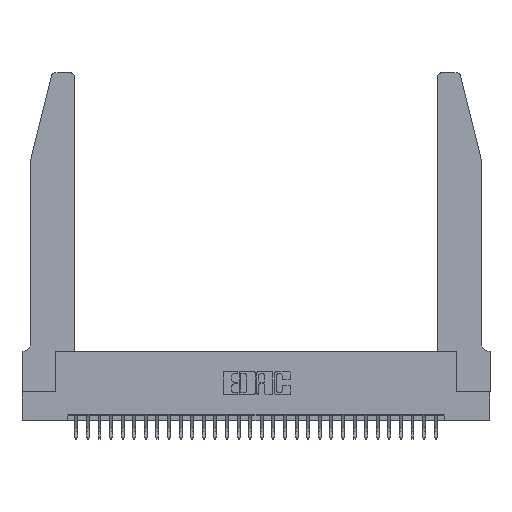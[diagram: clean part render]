
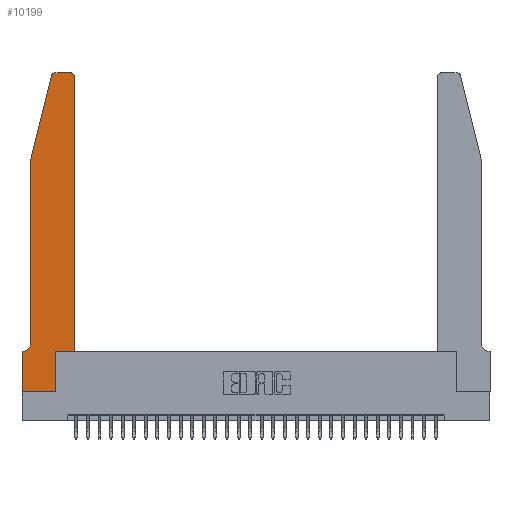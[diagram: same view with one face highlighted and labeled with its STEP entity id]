
A CAD part, top view. The second image highlights one B-rep face of the part: STEP entity #10199.
In plain terms, the highlighted planar face has unit normal (0, 0, 1).
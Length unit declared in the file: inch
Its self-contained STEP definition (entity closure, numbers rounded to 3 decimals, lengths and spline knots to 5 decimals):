
#533 = VECTOR ( 'NONE', #2375, 39.37008 ) ;
#574 = CARTESIAN_POINT ( 'NONE',  ( 0.0755, 0.42, 0.37 ) ) ;
#1327 = DIRECTION ( 'NONE',  ( 0., 1., 0. ) ) ;
#1335 = ORIENTED_EDGE ( 'NONE', *, *, #5731, .T. ) ;
#1471 = CARTESIAN_POINT ( 'NONE',  ( 0.2865, 0., 0.37 ) ) ;
#2073 = CARTESIAN_POINT ( 'NONE',  ( 0.4205, 2.72, 0.37 ) ) ;
#2176 = DIRECTION ( 'NONE',  ( 1., 0., 0. ) ) ;
#2247 = VECTOR ( 'NONE', #13660, 39.37008 ) ;
#2375 = DIRECTION ( 'NONE',  ( -1., 0., 0. ) ) ;
#2538 = EDGE_CURVE ( 'NONE', #26263, #22320, #18626, .T. ) ;
#2676 = VERTEX_POINT ( 'NONE', #9555 ) ;
#2763 = EDGE_CURVE ( 'NONE', #28510, #29235, #20082, .T. ) ;
#2786 = CARTESIAN_POINT ( 'NONE',  ( 0.2865, 0.35, 0.37 ) ) ;
#2855 = DIRECTION ( 'NONE',  ( 0., 0., -1. ) ) ;
#3597 = DIRECTION ( 'NONE',  ( 0., 0., 1. ) ) ;
#4156 = ORIENTED_EDGE ( 'NONE', *, *, #24620, .T. ) ;
#4180 = DIRECTION ( 'NONE',  ( 0., -1., 0. ) ) ;
#4250 = CIRCLE ( 'NONE', #20334, 0.07 ) ;
#4786 = AXIS2_PLACEMENT_3D ( 'NONE', #2073, #19172, #2176 ) ;
#4988 = VERTEX_POINT ( 'NONE', #8752 ) ;
#5173 = EDGE_CURVE ( 'NONE', #7477, #20418, #11264, .T. ) ;
#5637 = VERTEX_POINT ( 'NONE', #574 ) ;
#5731 = EDGE_CURVE ( 'NONE', #23783, #26263, #29848, .T. ) ;
#6413 = ORIENTED_EDGE ( 'NONE', *, *, #5173, .T. ) ;
#6653 = FACE_OUTER_BOUND ( 'NONE', #22145, .T. ) ;
#7132 = DIRECTION ( 'NONE',  ( 0., 0., 1. ) ) ;
#7250 = DIRECTION ( 'NONE',  ( -1., 0., 0. ) ) ;
#7477 = VERTEX_POINT ( 'NONE', #23795 ) ;
#7527 = ORIENTED_EDGE ( 'NONE', *, *, #22625, .T. ) ;
#7638 = CARTESIAN_POINT ( 'NONE',  ( 0.0055, 0.42, 0.37 ) ) ;
#8357 = CARTESIAN_POINT ( 'NONE',  ( 0.0755, 2., 0.37 ) ) ;
#8752 = CARTESIAN_POINT ( 'NONE',  ( 0.0055, 0.35, 0.37 ) ) ;
#8838 = EDGE_CURVE ( 'NONE', #5637, #4988, #4250, .T. ) ;
#9555 = CARTESIAN_POINT ( 'NONE',  ( 0.284, 2.75, 0.37 ) ) ;
#9731 = VECTOR ( 'NONE', #10140, 39.37008 ) ;
#10005 = CARTESIAN_POINT ( 'NONE',  ( 0.284, 2.72, 0.37 ) ) ;
#10140 = DIRECTION ( 'NONE',  ( 1., 0., 0. ) ) ;
#10199 = ADVANCED_FACE ( 'NONE', ( #6653 ), #18576, .T. ) ;
#10532 = VECTOR ( 'NONE', #13680, 39.37008 ) ;
#10593 = ORIENTED_EDGE ( 'NONE', *, *, #11465, .T. ) ;
#11264 = LINE ( 'NONE', #26016, #16211 ) ;
#11465 = EDGE_CURVE ( 'NONE', #20418, #17329, #13440, .T. ) ;
#11520 = LINE ( 'NONE', #19045, #19884 ) ;
#13440 = LINE ( 'NONE', #16291, #14199 ) ;
#13589 = CARTESIAN_POINT ( 'NONE',  ( 0., 0.35, 0.37 ) ) ;
#13660 = DIRECTION ( 'NONE',  ( -0.239, -0.971, 0. ) ) ;
#13664 = CIRCLE ( 'NONE', #4786, 0.03 ) ;
#13680 = DIRECTION ( 'NONE',  ( 0., -1., 0. ) ) ;
#13976 = EDGE_CURVE ( 'NONE', #22320, #15473, #13664, .T. ) ;
#14199 = VECTOR ( 'NONE', #28607, 39.37008 ) ;
#14656 = EDGE_CURVE ( 'NONE', #2676, #28510, #14735, .T. ) ;
#14735 = CIRCLE ( 'NONE', #31254, 0.03 ) ;
#14776 = VECTOR ( 'NONE', #1327, 39.37008 ) ;
#15473 = VERTEX_POINT ( 'NONE', #25119 ) ;
#16211 = VECTOR ( 'NONE', #4180, 39.37008 ) ;
#16291 = CARTESIAN_POINT ( 'NONE',  ( 0., 0., 0.37 ) ) ;
#17114 = VECTOR ( 'NONE', #28820, 39.37008 ) ;
#17196 = DIRECTION ( 'NONE',  ( -1., 0., 0. ) ) ;
#17244 = ORIENTED_EDGE ( 'NONE', *, *, #13976, .T. ) ;
#17255 = ORIENTED_EDGE ( 'NONE', *, *, #14656, .T. ) ;
#17329 = VERTEX_POINT ( 'NONE', #1471 ) ;
#17767 = CARTESIAN_POINT ( 'NONE',  ( 0.4505, 0.35, 0.37 ) ) ;
#18576 = PLANE ( 'NONE',  #26230 ) ;
#18626 = LINE ( 'NONE', #17767, #14776 ) ;
#18645 = ORIENTED_EDGE ( 'NONE', *, *, #2538, .T. ) ;
#19045 = CARTESIAN_POINT ( 'NONE',  ( 0.0755, 0.35, 0.37 ) ) ;
#19156 = CARTESIAN_POINT ( 'NONE',  ( 0.2865, 0.35, 0.37 ) ) ;
#19172 = DIRECTION ( 'NONE',  ( 0., 0., 1. ) ) ;
#19884 = VECTOR ( 'NONE', #7250, 39.37008 ) ;
#20082 = LINE ( 'NONE', #24800, #2247 ) ;
#20212 = CARTESIAN_POINT ( 'NONE',  ( 0.4505, 0.35, 0.37 ) ) ;
#20334 = AXIS2_PLACEMENT_3D ( 'NONE', #7638, #2855, #17196 ) ;
#20418 = VERTEX_POINT ( 'NONE', #30352 ) ;
#22145 = EDGE_LOOP ( 'NONE', ( #28583, #17255, #30727, #4156, #23805, #7527, #6413, #10593, #26751, #1335, #18645, #17244 ) ) ;
#22216 = LINE ( 'NONE', #26547, #533 ) ;
#22320 = VERTEX_POINT ( 'NONE', #30072 ) ;
#22530 = CARTESIAN_POINT ( 'NONE',  ( 0.25487, 2.72718, 0.37 ) ) ;
#22625 = EDGE_CURVE ( 'NONE', #4988, #7477, #11520, .T. ) ;
#22703 = CARTESIAN_POINT ( 'NONE',  ( 0.0755, 2., 0.37 ) ) ;
#23783 = VERTEX_POINT ( 'NONE', #2786 ) ;
#23795 = CARTESIAN_POINT ( 'NONE',  ( 0., 0.35, 0.37 ) ) ;
#23805 = ORIENTED_EDGE ( 'NONE', *, *, #8838, .T. ) ;
#24620 = EDGE_CURVE ( 'NONE', #29235, #5637, #30692, .T. ) ;
#24800 = CARTESIAN_POINT ( 'NONE',  ( 0.0755, 2., 0.37 ) ) ;
#25119 = CARTESIAN_POINT ( 'NONE',  ( 0.4205, 2.75, 0.37 ) ) ;
#25940 = CARTESIAN_POINT ( 'NONE',  ( 0.4505, 0.35, 0.37 ) ) ;
#26016 = CARTESIAN_POINT ( 'NONE',  ( 0., 0., 0.37 ) ) ;
#26216 = LINE ( 'NONE', #19156, #17114 ) ;
#26230 = AXIS2_PLACEMENT_3D ( 'NONE', #13589, #3597, #30564 ) ;
#26263 = VERTEX_POINT ( 'NONE', #25940 ) ;
#26294 = EDGE_CURVE ( 'NONE', #15473, #2676, #22216, .T. ) ;
#26547 = CARTESIAN_POINT ( 'NONE',  ( 0.2605, 2.75, 0.37 ) ) ;
#26751 = ORIENTED_EDGE ( 'NONE', *, *, #28199, .T. ) ;
#28199 = EDGE_CURVE ( 'NONE', #17329, #23783, #26216, .T. ) ;
#28510 = VERTEX_POINT ( 'NONE', #22530 ) ;
#28583 = ORIENTED_EDGE ( 'NONE', *, *, #26294, .T. ) ;
#28607 = DIRECTION ( 'NONE',  ( 1., 0., 0. ) ) ;
#28820 = DIRECTION ( 'NONE',  ( 0., 1., 0. ) ) ;
#29012 = DIRECTION ( 'NONE',  ( 1., 0., 0. ) ) ;
#29235 = VERTEX_POINT ( 'NONE', #8357 ) ;
#29848 = LINE ( 'NONE', #20212, #9731 ) ;
#30072 = CARTESIAN_POINT ( 'NONE',  ( 0.4505, 2.72, 0.37 ) ) ;
#30352 = CARTESIAN_POINT ( 'NONE',  ( 0., 0., 0.37 ) ) ;
#30564 = DIRECTION ( 'NONE',  ( 1., 0., 0. ) ) ;
#30692 = LINE ( 'NONE', #22703, #10532 ) ;
#30727 = ORIENTED_EDGE ( 'NONE', *, *, #2763, .T. ) ;
#31254 = AXIS2_PLACEMENT_3D ( 'NONE', #10005, #7132, #29012 ) ;
